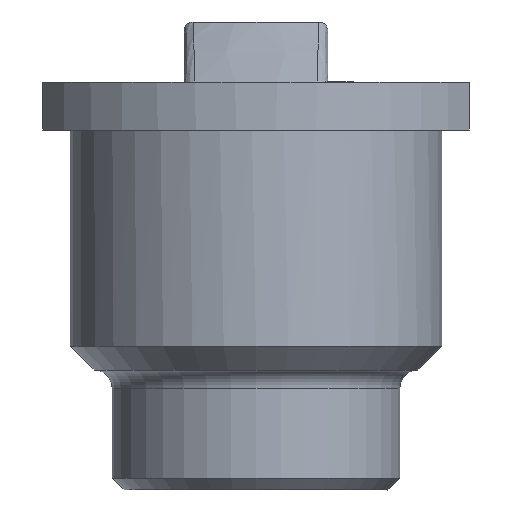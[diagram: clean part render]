
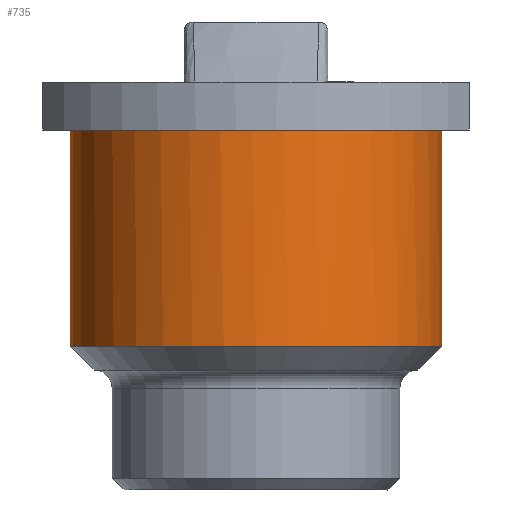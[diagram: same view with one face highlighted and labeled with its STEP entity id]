
A CAD part, front view. The second image highlights one B-rep face of the part: STEP entity #735.
In plain terms, the highlighted cylindrical face has radius 7.75 mm (diameter 15.5 mm), a full revolution.
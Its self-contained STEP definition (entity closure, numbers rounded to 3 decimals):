
#46=CIRCLE('',#796,7.75);
#48=CIRCLE('',#798,7.75);
#54=CIRCLE('',#805,7.75);
#55=CIRCLE('',#806,7.75);
#56=CIRCLE('',#807,7.75);
#57=CIRCLE('',#808,7.75);
#58=CIRCLE('',#809,7.75);
#92=CYLINDRICAL_SURFACE('',#804,7.75);
#112=FACE_OUTER_BOUND('',#156,.T.);
#156=EDGE_LOOP('',(#543,#544,#545,#546,#547,#548,#549,#550,#551,#552,#553,
#554,#555));
#207=LINE('',#1139,#260);
#210=LINE('',#1148,#263);
#215=LINE('',#1158,#268);
#218=LINE('',#1165,#271);
#226=LINE('',#1249,#279);
#260=VECTOR('',#899,10.);
#263=VECTOR('',#908,10.);
#268=VECTOR('',#915,10.);
#271=VECTOR('',#920,10.);
#279=VECTOR('',#952,7.75);
#312=VERTEX_POINT('',#1136);
#313=VERTEX_POINT('',#1138);
#315=VERTEX_POINT('',#1146);
#316=VERTEX_POINT('',#1147);
#319=VERTEX_POINT('',#1155);
#320=VERTEX_POINT('',#1157);
#322=VERTEX_POINT('',#1163);
#323=VERTEX_POINT('',#1164);
#336=VERTEX_POINT('',#1246);
#337=VERTEX_POINT('',#1248);
#338=VERTEX_POINT('',#1250);
#387=EDGE_CURVE('',#312,#313,#207,.T.);
#391=EDGE_CURVE('',#315,#316,#210,.T.);
#396=EDGE_CURVE('',#319,#320,#215,.T.);
#399=EDGE_CURVE('',#322,#323,#218,.T.);
#403=EDGE_CURVE('',#312,#323,#46,.T.);
#405=EDGE_CURVE('',#315,#320,#48,.T.);
#417=EDGE_CURVE('',#313,#319,#54,.T.);
#418=EDGE_CURVE('',#336,#322,#55,.T.);
#419=EDGE_CURVE('',#336,#337,#226,.T.);
#420=EDGE_CURVE('',#338,#337,#56,.T.);
#421=EDGE_CURVE('',#337,#338,#57,.T.);
#422=EDGE_CURVE('',#316,#336,#58,.T.);
#543=ORIENTED_EDGE('',*,*,#391,.F.);
#544=ORIENTED_EDGE('',*,*,#405,.T.);
#545=ORIENTED_EDGE('',*,*,#396,.F.);
#546=ORIENTED_EDGE('',*,*,#417,.F.);
#547=ORIENTED_EDGE('',*,*,#387,.F.);
#548=ORIENTED_EDGE('',*,*,#403,.T.);
#549=ORIENTED_EDGE('',*,*,#399,.F.);
#550=ORIENTED_EDGE('',*,*,#418,.F.);
#551=ORIENTED_EDGE('',*,*,#419,.T.);
#552=ORIENTED_EDGE('',*,*,#420,.F.);
#553=ORIENTED_EDGE('',*,*,#421,.F.);
#554=ORIENTED_EDGE('',*,*,#419,.F.);
#555=ORIENTED_EDGE('',*,*,#422,.F.);
#735=ADVANCED_FACE('',(#112),#92,.T.);
#796=AXIS2_PLACEMENT_3D('',#1172,#926,#927);
#798=AXIS2_PLACEMENT_3D('',#1174,#930,#931);
#804=AXIS2_PLACEMENT_3D('',#1244,#946,#947);
#805=AXIS2_PLACEMENT_3D('',#1245,#948,#949);
#806=AXIS2_PLACEMENT_3D('',#1247,#950,#951);
#807=AXIS2_PLACEMENT_3D('',#1251,#953,#954);
#808=AXIS2_PLACEMENT_3D('',#1252,#955,#956);
#809=AXIS2_PLACEMENT_3D('',#1253,#957,#958);
#899=DIRECTION('',(0.,0.,-1.));
#908=DIRECTION('',(0.,0.,-1.));
#915=DIRECTION('',(0.,0.,1.));
#920=DIRECTION('',(0.,0.,1.));
#926=DIRECTION('center_axis',(0.,0.,-1.));
#927=DIRECTION('ref_axis',(1.,0.,0.));
#930=DIRECTION('center_axis',(0.,0.,-1.));
#931=DIRECTION('ref_axis',(1.,0.,0.));
#946=DIRECTION('center_axis',(0.,0.,1.));
#947=DIRECTION('ref_axis',(1.,0.,0.));
#948=DIRECTION('center_axis',(0.,0.,1.));
#949=DIRECTION('ref_axis',(1.,0.,0.));
#950=DIRECTION('center_axis',(0.,0.,1.));
#951=DIRECTION('ref_axis',(1.,0.,0.));
#952=DIRECTION('',(0.,0.,-1.));
#953=DIRECTION('center_axis',(0.,0.,-1.));
#954=DIRECTION('ref_axis',(-1.,0.,0.));
#955=DIRECTION('center_axis',(0.,0.,-1.));
#956=DIRECTION('ref_axis',(-1.,0.,0.));
#957=DIRECTION('center_axis',(0.,0.,1.));
#958=DIRECTION('ref_axis',(1.,0.,0.));
#1136=CARTESIAN_POINT('',(1.075,7.675,7.));
#1138=CARTESIAN_POINT('',(1.075,7.675,5.));
#1139=CARTESIAN_POINT('',(1.075,7.675,4.8));
#1146=CARTESIAN_POINT('',(-1.825,7.532,7.));
#1147=CARTESIAN_POINT('',(-1.825,7.532,5.));
#1148=CARTESIAN_POINT('',(-1.825,7.532,4.8));
#1155=CARTESIAN_POINT('',(-1.075,7.675,5.));
#1157=CARTESIAN_POINT('',(-1.075,7.675,7.));
#1158=CARTESIAN_POINT('',(-1.075,7.675,4.8));
#1163=CARTESIAN_POINT('',(1.825,7.532,5.));
#1164=CARTESIAN_POINT('',(1.825,7.532,7.));
#1165=CARTESIAN_POINT('',(1.825,7.532,4.8));
#1172=CARTESIAN_POINT('Origin',(0.,0.,7.));
#1174=CARTESIAN_POINT('Origin',(0.,0.,7.));
#1244=CARTESIAN_POINT('Origin',(0.,0.,0.));
#1245=CARTESIAN_POINT('Origin',(0.,0.,5.));
#1246=CARTESIAN_POINT('',(-7.75,0.,5.));
#1247=CARTESIAN_POINT('Origin',(0.,0.,5.));
#1248=CARTESIAN_POINT('',(-7.75,0.,-4.));
#1249=CARTESIAN_POINT('',(-7.75,0.,0.));
#1250=CARTESIAN_POINT('',(7.75,0.,-4.));
#1251=CARTESIAN_POINT('Origin',(0.,0.,-4.));
#1252=CARTESIAN_POINT('Origin',(0.,0.,-4.));
#1253=CARTESIAN_POINT('Origin',(0.,0.,5.));
